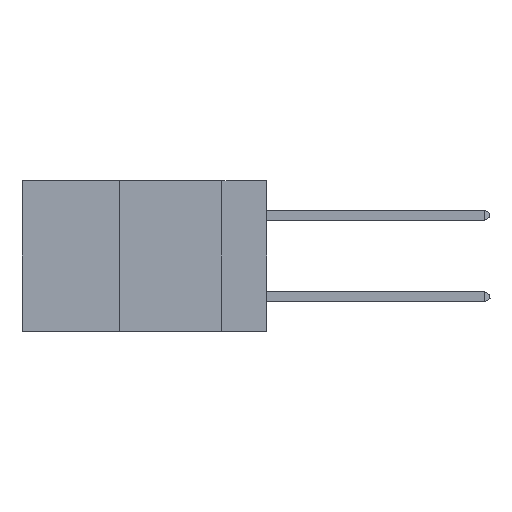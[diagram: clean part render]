
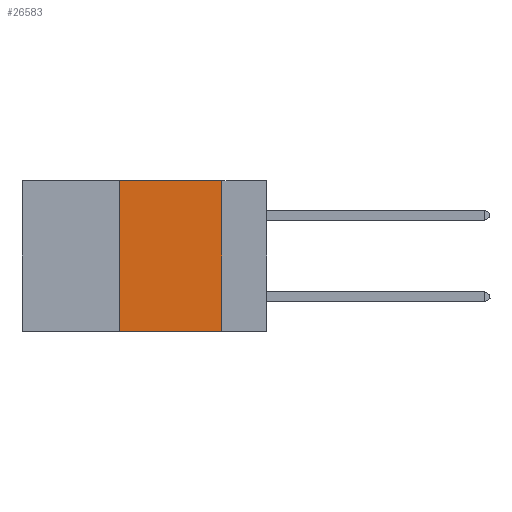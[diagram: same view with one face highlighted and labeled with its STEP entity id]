
A CAD part, left-side view. The second image highlights one B-rep face of the part: STEP entity #26583.
In plain terms, the highlighted planar face has unit normal (-1, 0, 0).
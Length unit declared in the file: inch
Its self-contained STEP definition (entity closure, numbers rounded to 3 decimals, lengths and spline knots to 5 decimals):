
#417 = DIRECTION ( 'NONE',  ( 0., -1., 0. ) ) ;
#554 = VECTOR ( 'NONE', #36534, 39.37008 ) ;
#1972 = VERTEX_POINT ( 'NONE', #14505 ) ;
#2058 = LINE ( 'NONE', #31533, #20287 ) ;
#2132 = VERTEX_POINT ( 'NONE', #3561 ) ;
#3561 = CARTESIAN_POINT ( 'NONE',  ( 0., 0.11, 0. ) ) ;
#3681 = LINE ( 'NONE', #12171, #33613 ) ;
#5177 = FACE_OUTER_BOUND ( 'NONE', #32586, .T. ) ;
#5601 = DIRECTION ( 'NONE',  ( 0., -1., 0. ) ) ;
#5836 = CARTESIAN_POINT ( 'NONE',  ( 0., 0.36, -0.37 ) ) ;
#7325 = VECTOR ( 'NONE', #24027, 39.37008 ) ;
#8321 = CARTESIAN_POINT ( 'NONE',  ( 0., 0.36, 0. ) ) ;
#9757 = CARTESIAN_POINT ( 'NONE',  ( 0., 0.6, 0. ) ) ;
#12171 = CARTESIAN_POINT ( 'NONE',  ( 0., 0.6, -0.37 ) ) ;
#14363 = EDGE_CURVE ( 'NONE', #36540, #16290, #23781, .T. ) ;
#14505 = CARTESIAN_POINT ( 'NONE',  ( 0., 0.11, -0.37 ) ) ;
#15714 = DIRECTION ( 'NONE',  ( 0., 0., -1. ) ) ;
#15813 = EDGE_CURVE ( 'NONE', #36540, #1972, #3681, .T. ) ;
#16290 = VERTEX_POINT ( 'NONE', #8321 ) ;
#17014 = AXIS2_PLACEMENT_3D ( 'NONE', #9757, #32918, #15714 ) ;
#20287 = VECTOR ( 'NONE', #5601, 39.37008 ) ;
#22175 = CARTESIAN_POINT ( 'NONE',  ( 0., 0.36, 0. ) ) ;
#22386 = ORIENTED_EDGE ( 'NONE', *, *, #24409, .F. ) ;
#23566 = LINE ( 'NONE', #29839, #7325 ) ;
#23781 = LINE ( 'NONE', #22175, #554 ) ;
#24027 = DIRECTION ( 'NONE',  ( 0., 0., -1. ) ) ;
#24409 = EDGE_CURVE ( 'NONE', #16290, #2132, #2058, .T. ) ;
#26583 = ADVANCED_FACE ( 'NONE', ( #5177 ), #27097, .F. ) ;
#26675 = ORIENTED_EDGE ( 'NONE', *, *, #15813, .T. ) ;
#27097 = PLANE ( 'NONE',  #17014 ) ;
#29138 = ORIENTED_EDGE ( 'NONE', *, *, #32411, .F. ) ;
#29839 = CARTESIAN_POINT ( 'NONE',  ( 0., 0.11, 0. ) ) ;
#31533 = CARTESIAN_POINT ( 'NONE',  ( 0., 0.6, 0. ) ) ;
#32411 = EDGE_CURVE ( 'NONE', #2132, #1972, #23566, .T. ) ;
#32586 = EDGE_LOOP ( 'NONE', ( #29138, #22386, #36145, #26675 ) ) ;
#32918 = DIRECTION ( 'NONE',  ( 1., 0., 0. ) ) ;
#33613 = VECTOR ( 'NONE', #417, 39.37008 ) ;
#36145 = ORIENTED_EDGE ( 'NONE', *, *, #14363, .F. ) ;
#36534 = DIRECTION ( 'NONE',  ( 0., 0., 1. ) ) ;
#36540 = VERTEX_POINT ( 'NONE', #5836 ) ;
